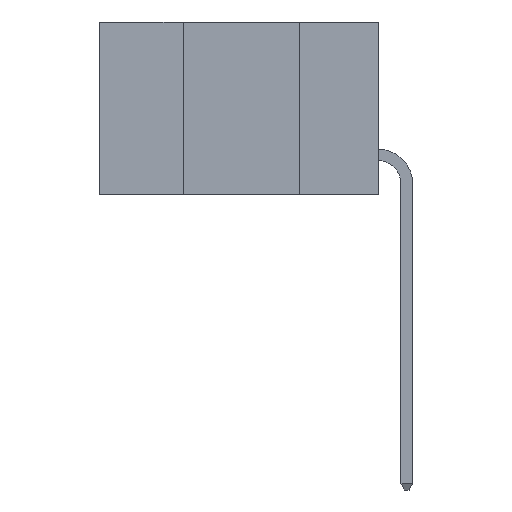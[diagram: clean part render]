
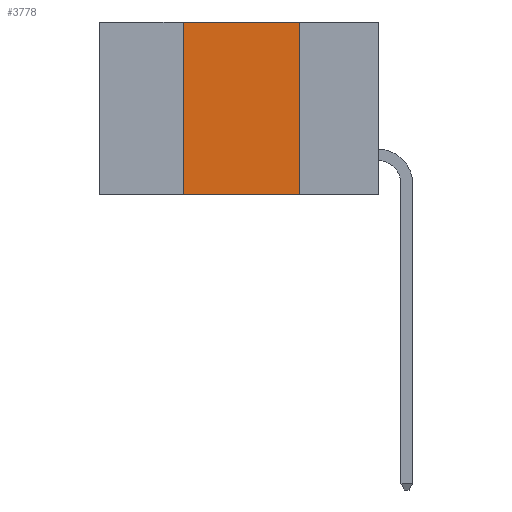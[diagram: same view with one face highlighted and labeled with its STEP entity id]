
A CAD part, left-side view. The second image highlights one B-rep face of the part: STEP entity #3778.
In plain terms, the highlighted planar face has unit normal (-1, 0, 0).
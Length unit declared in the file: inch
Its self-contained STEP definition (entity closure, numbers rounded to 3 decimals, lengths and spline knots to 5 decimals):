
#60 = FACE_OUTER_BOUND ( 'NONE', #11136, .T. ) ;
#373 = LINE ( 'NONE', #3357, #11605 ) ;
#476 = ORIENTED_EDGE ( 'NONE', *, *, #4125, .F. ) ;
#876 = EDGE_CURVE ( 'NONE', #3940, #1130, #11040, .T. ) ;
#1130 = VERTEX_POINT ( 'NONE', #13704 ) ;
#1326 = DIRECTION ( 'NONE',  ( 0., -1., 0. ) ) ;
#1686 = ORIENTED_EDGE ( 'NONE', *, *, #1785, .F. ) ;
#1785 = EDGE_CURVE ( 'NONE', #3831, #3610, #7038, .T. ) ;
#2004 = CARTESIAN_POINT ( 'NONE',  ( 0., 0.42, -0.37 ) ) ;
#2801 = DIRECTION ( 'NONE',  ( 1., 0., 0. ) ) ;
#3357 = CARTESIAN_POINT ( 'NONE',  ( 0., 0.17, -0.37 ) ) ;
#3610 = VERTEX_POINT ( 'NONE', #13399 ) ;
#3778 = ADVANCED_FACE ( 'NONE', ( #60 ), #7074, .F. ) ;
#3831 = VERTEX_POINT ( 'NONE', #13783 ) ;
#3940 = VERTEX_POINT ( 'NONE', #2004 ) ;
#4125 = EDGE_CURVE ( 'NONE', #3610, #1130, #373, .T. ) ;
#4179 = DIRECTION ( 'NONE',  ( 0., 0., 1. ) ) ;
#4357 = ORIENTED_EDGE ( 'NONE', *, *, #876, .T. ) ;
#4392 = DIRECTION ( 'NONE',  ( 0., 0., -1. ) ) ;
#7038 = LINE ( 'NONE', #13270, #8964 ) ;
#7074 = PLANE ( 'NONE',  #7250 ) ;
#7250 = AXIS2_PLACEMENT_3D ( 'NONE', #9320, #2801, #10403 ) ;
#8517 = LINE ( 'NONE', #10725, #9545 ) ;
#8964 = VECTOR ( 'NONE', #1326, 39.37008 ) ;
#9014 = ORIENTED_EDGE ( 'NONE', *, *, #13242, .F. ) ;
#9320 = CARTESIAN_POINT ( 'NONE',  ( 0., 0.6, 0. ) ) ;
#9545 = VECTOR ( 'NONE', #4179, 39.37008 ) ;
#9705 = CARTESIAN_POINT ( 'NONE',  ( 0., 0.6, -0.37 ) ) ;
#10009 = DIRECTION ( 'NONE',  ( 0., -1., 0. ) ) ;
#10403 = DIRECTION ( 'NONE',  ( 0., 0., -1. ) ) ;
#10725 = CARTESIAN_POINT ( 'NONE',  ( 0., 0.42, -0.37 ) ) ;
#11040 = LINE ( 'NONE', #9705, #13588 ) ;
#11136 = EDGE_LOOP ( 'NONE', ( #476, #1686, #9014, #4357 ) ) ;
#11605 = VECTOR ( 'NONE', #4392, 39.37008 ) ;
#13242 = EDGE_CURVE ( 'NONE', #3940, #3831, #8517, .T. ) ;
#13270 = CARTESIAN_POINT ( 'NONE',  ( 0., 0.6, 0. ) ) ;
#13399 = CARTESIAN_POINT ( 'NONE',  ( 0., 0.17, 0. ) ) ;
#13588 = VECTOR ( 'NONE', #10009, 39.37008 ) ;
#13704 = CARTESIAN_POINT ( 'NONE',  ( 0., 0.17, -0.37 ) ) ;
#13783 = CARTESIAN_POINT ( 'NONE',  ( 0., 0.42, 0. ) ) ;
